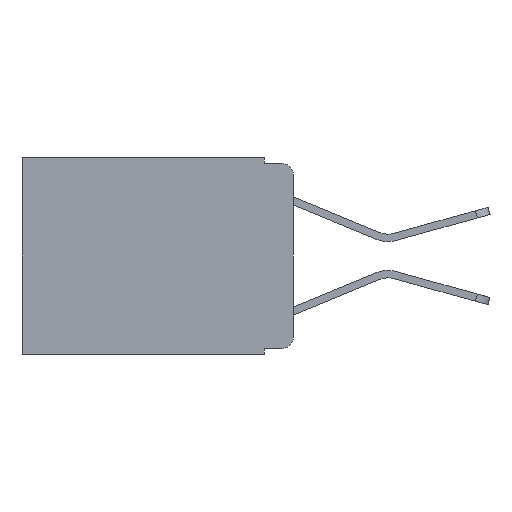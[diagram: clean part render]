
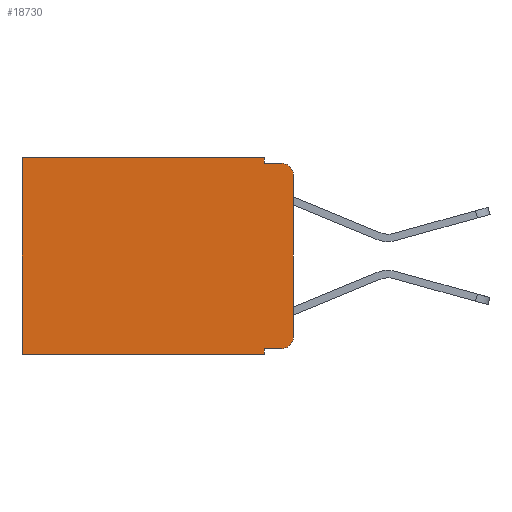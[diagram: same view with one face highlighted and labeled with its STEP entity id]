
A CAD part, left-side view. The second image highlights one B-rep face of the part: STEP entity #18730.
In plain terms, the highlighted planar face has unit normal (-1, 0, 0).
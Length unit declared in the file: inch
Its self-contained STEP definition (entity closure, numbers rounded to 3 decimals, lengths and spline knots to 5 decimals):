
#131 = AXIS2_PLACEMENT_3D ( 'NONE', #9893, #11806, #317 ) ;
#217 = CARTESIAN_POINT ( 'NONE',  ( 0.298, 0.051, 0. ) ) ;
#317 = DIRECTION ( 'NONE',  ( 0., 0., -1. ) ) ;
#516 = CARTESIAN_POINT ( 'NONE',  ( 0.298, 0.02, -0.333 ) ) ;
#608 = CARTESIAN_POINT ( 'NONE',  ( 0.298, 0.051, -0.333 ) ) ;
#925 = EDGE_CURVE ( 'NONE', #14458, #6351, #8248, .T. ) ;
#1068 = EDGE_CURVE ( 'NONE', #14971, #19519, #2807, .T. ) ;
#1289 = VECTOR ( 'NONE', #5438, 39.37008 ) ;
#1507 = VERTEX_POINT ( 'NONE', #608 ) ;
#1537 = VECTOR ( 'NONE', #9656, 39.37008 ) ;
#1672 = DIRECTION ( 'NONE',  ( 0., 0., -1. ) ) ;
#1714 = DIRECTION ( 'NONE',  ( -1., 0., 0. ) ) ;
#1909 = CIRCLE ( 'NONE', #15973, 0.02 ) ;
#2076 = CARTESIAN_POINT ( 'NONE',  ( 0.298, 0., 0. ) ) ;
#2807 = LINE ( 'NONE', #4819, #12981 ) ;
#2965 = CIRCLE ( 'NONE', #4427, 0.02 ) ;
#3409 = ORIENTED_EDGE ( 'NONE', *, *, #8807, .F. ) ;
#3649 = VECTOR ( 'NONE', #13040, 39.37008 ) ;
#4427 = AXIS2_PLACEMENT_3D ( 'NONE', #13176, #1714, #15055 ) ;
#4819 = CARTESIAN_POINT ( 'NONE',  ( 0.298, 0.051, -0.01 ) ) ;
#4945 = EDGE_CURVE ( 'NONE', #15825, #19519, #2965, .T. ) ;
#5062 = DIRECTION ( 'NONE',  ( 0., -1., 0. ) ) ;
#5438 = DIRECTION ( 'NONE',  ( 0., 1., 0. ) ) ;
#5528 = ORIENTED_EDGE ( 'NONE', *, *, #4945, .T. ) ;
#5741 = CARTESIAN_POINT ( 'NONE',  ( 0.298, 0., 0. ) ) ;
#6351 = VERTEX_POINT ( 'NONE', #15318 ) ;
#6697 = LINE ( 'NONE', #9727, #1537 ) ;
#6767 = VERTEX_POINT ( 'NONE', #13102 ) ;
#7752 = VECTOR ( 'NONE', #15403, 39.37008 ) ;
#8023 = EDGE_CURVE ( 'NONE', #15095, #22915, #1909, .T. ) ;
#8248 = LINE ( 'NONE', #9511, #1289 ) ;
#8807 = EDGE_CURVE ( 'NONE', #15825, #22915, #23742, .T. ) ;
#9272 = EDGE_CURVE ( 'NONE', #1507, #15095, #14360, .T. ) ;
#9292 = CARTESIAN_POINT ( 'NONE',  ( 0.298, 0.051, -0.333 ) ) ;
#9511 = CARTESIAN_POINT ( 'NONE',  ( 0.298, 0., -0.343 ) ) ;
#9656 = DIRECTION ( 'NONE',  ( 0., 0., -1. ) ) ;
#9727 = CARTESIAN_POINT ( 'NONE',  ( 0.298, 0.473, 0. ) ) ;
#9785 = VERTEX_POINT ( 'NONE', #18444 ) ;
#9893 = CARTESIAN_POINT ( 'NONE',  ( 0.298, 0., 0. ) ) ;
#10587 = CARTESIAN_POINT ( 'NONE',  ( 0.298, 0.02, -0.01 ) ) ;
#10636 = CARTESIAN_POINT ( 'NONE',  ( 0.298, 0., -0.313 ) ) ;
#11098 = CARTESIAN_POINT ( 'NONE',  ( 0.298, 0.02, -0.313 ) ) ;
#11215 = LINE ( 'NONE', #217, #16213 ) ;
#11236 = CARTESIAN_POINT ( 'NONE',  ( 0.298, 0.051, 0. ) ) ;
#11514 = ORIENTED_EDGE ( 'NONE', *, *, #18179, .T. ) ;
#11806 = DIRECTION ( 'NONE',  ( 1., 0., 0. ) ) ;
#11831 = ORIENTED_EDGE ( 'NONE', *, *, #8023, .T. ) ;
#12689 = ORIENTED_EDGE ( 'NONE', *, *, #14363, .F. ) ;
#12981 = VECTOR ( 'NONE', #5062, 39.37008 ) ;
#13009 = DIRECTION ( 'NONE',  ( 0., 0., -1. ) ) ;
#13040 = DIRECTION ( 'NONE',  ( 0., -1., 0. ) ) ;
#13102 = CARTESIAN_POINT ( 'NONE',  ( 0.298, 0.473, 0. ) ) ;
#13176 = CARTESIAN_POINT ( 'NONE',  ( 0.298, 0.02, -0.03 ) ) ;
#13611 = DIRECTION ( 'NONE',  ( 0., 0., -1. ) ) ;
#14019 = VECTOR ( 'NONE', #1672, 39.37008 ) ;
#14360 = LINE ( 'NONE', #9292, #3649 ) ;
#14363 = EDGE_CURVE ( 'NONE', #1507, #14458, #11215, .T. ) ;
#14458 = VERTEX_POINT ( 'NONE', #21298 ) ;
#14485 = EDGE_LOOP ( 'NONE', ( #3409, #5528, #19173, #20329, #11514, #16479, #23214, #12689, #18600, #11831 ) ) ;
#14971 = VERTEX_POINT ( 'NONE', #15376 ) ;
#15055 = DIRECTION ( 'NONE',  ( 0., 0., -1. ) ) ;
#15095 = VERTEX_POINT ( 'NONE', #516 ) ;
#15318 = CARTESIAN_POINT ( 'NONE',  ( 0.298, 0.473, -0.343 ) ) ;
#15376 = CARTESIAN_POINT ( 'NONE',  ( 0.298, 0.051, -0.01 ) ) ;
#15403 = DIRECTION ( 'NONE',  ( 0., 1., 0. ) ) ;
#15619 = EDGE_CURVE ( 'NONE', #6767, #6351, #6697, .T. ) ;
#15825 = VERTEX_POINT ( 'NONE', #18537 ) ;
#15973 = AXIS2_PLACEMENT_3D ( 'NONE', #11098, #24169, #13009 ) ;
#16213 = VECTOR ( 'NONE', #13611, 39.37008 ) ;
#16479 = ORIENTED_EDGE ( 'NONE', *, *, #15619, .T. ) ;
#17812 = LINE ( 'NONE', #2076, #7752 ) ;
#18179 = EDGE_CURVE ( 'NONE', #9785, #6767, #17812, .T. ) ;
#18444 = CARTESIAN_POINT ( 'NONE',  ( 0.298, 0.051, 0. ) ) ;
#18537 = CARTESIAN_POINT ( 'NONE',  ( 0.298, 0., -0.03 ) ) ;
#18600 = ORIENTED_EDGE ( 'NONE', *, *, #9272, .T. ) ;
#18730 = ADVANCED_FACE ( 'NONE', ( #20982 ), #21149, .F. ) ;
#18827 = VECTOR ( 'NONE', #24460, 39.37008 ) ;
#19012 = LINE ( 'NONE', #11236, #14019 ) ;
#19173 = ORIENTED_EDGE ( 'NONE', *, *, #1068, .F. ) ;
#19519 = VERTEX_POINT ( 'NONE', #10587 ) ;
#20329 = ORIENTED_EDGE ( 'NONE', *, *, #20649, .F. ) ;
#20649 = EDGE_CURVE ( 'NONE', #9785, #14971, #19012, .T. ) ;
#20982 = FACE_OUTER_BOUND ( 'NONE', #14485, .T. ) ;
#21149 = PLANE ( 'NONE',  #131 ) ;
#21298 = CARTESIAN_POINT ( 'NONE',  ( 0.298, 0.051, -0.343 ) ) ;
#22915 = VERTEX_POINT ( 'NONE', #10636 ) ;
#23214 = ORIENTED_EDGE ( 'NONE', *, *, #925, .F. ) ;
#23742 = LINE ( 'NONE', #5741, #18827 ) ;
#24169 = DIRECTION ( 'NONE',  ( -1., 0., 0. ) ) ;
#24460 = DIRECTION ( 'NONE',  ( 0., 0., -1. ) ) ;
